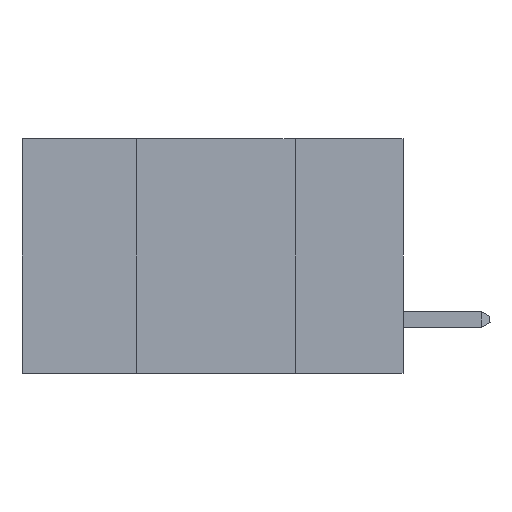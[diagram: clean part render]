
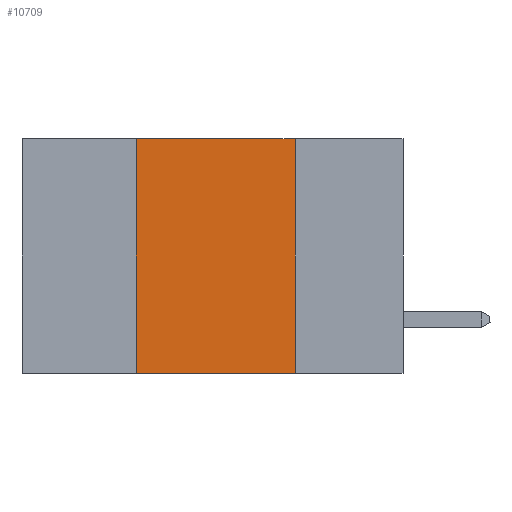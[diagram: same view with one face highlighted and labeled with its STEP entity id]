
A CAD part, left-side view. The second image highlights one B-rep face of the part: STEP entity #10709.
In plain terms, the highlighted planar face has unit normal (-1, 0, 0).
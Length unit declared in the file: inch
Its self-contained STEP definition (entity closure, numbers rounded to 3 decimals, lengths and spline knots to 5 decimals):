
#49 = VECTOR ( 'NONE', #16584, 39.37008 ) ;
#674 = CARTESIAN_POINT ( 'NONE',  ( 0., 0.42, -0.37 ) ) ;
#1449 = DIRECTION ( 'NONE',  ( 0., 0., -1. ) ) ;
#2698 = ORIENTED_EDGE ( 'NONE', *, *, #3617, .F. ) ;
#2763 = AXIS2_PLACEMENT_3D ( 'NONE', #7770, #7904, #1449 ) ;
#3161 = FACE_OUTER_BOUND ( 'NONE', #6307, .T. ) ;
#3617 = EDGE_CURVE ( 'NONE', #12747, #12285, #8369, .T. ) ;
#3653 = VECTOR ( 'NONE', #14696, 39.37008 ) ;
#5857 = CARTESIAN_POINT ( 'NONE',  ( 0., 0.17, 0. ) ) ;
#6307 = EDGE_LOOP ( 'NONE', ( #6329, #19401, #2698, #15257 ) ) ;
#6329 = ORIENTED_EDGE ( 'NONE', *, *, #15482, .F. ) ;
#6405 = CARTESIAN_POINT ( 'NONE',  ( 0., 0.6, 0. ) ) ;
#6597 = DIRECTION ( 'NONE',  ( 0., -1., 0. ) ) ;
#6686 = CARTESIAN_POINT ( 'NONE',  ( 0., 0.42, 0. ) ) ;
#7086 = CARTESIAN_POINT ( 'NONE',  ( 0., 0.17, -0.37 ) ) ;
#7698 = VECTOR ( 'NONE', #16196, 39.37008 ) ;
#7770 = CARTESIAN_POINT ( 'NONE',  ( 0., 0.6, 0. ) ) ;
#7904 = DIRECTION ( 'NONE',  ( 1., 0., 0. ) ) ;
#7906 = EDGE_CURVE ( 'NONE', #12285, #15036, #14683, .T. ) ;
#8369 = LINE ( 'NONE', #6686, #3653 ) ;
#10099 = LINE ( 'NONE', #11348, #17526 ) ;
#10709 = ADVANCED_FACE ( 'NONE', ( #3161 ), #20320, .F. ) ;
#11348 = CARTESIAN_POINT ( 'NONE',  ( 0., 0.6, -0.37 ) ) ;
#12285 = VERTEX_POINT ( 'NONE', #19545 ) ;
#12747 = VERTEX_POINT ( 'NONE', #674 ) ;
#13448 = VERTEX_POINT ( 'NONE', #7086 ) ;
#14511 = LINE ( 'NONE', #18129, #49 ) ;
#14683 = LINE ( 'NONE', #6405, #7698 ) ;
#14696 = DIRECTION ( 'NONE',  ( 0., 0., 1. ) ) ;
#15036 = VERTEX_POINT ( 'NONE', #5857 ) ;
#15257 = ORIENTED_EDGE ( 'NONE', *, *, #20266, .T. ) ;
#15482 = EDGE_CURVE ( 'NONE', #15036, #13448, #14511, .T. ) ;
#16196 = DIRECTION ( 'NONE',  ( 0., -1., 0. ) ) ;
#16584 = DIRECTION ( 'NONE',  ( 0., 0., -1. ) ) ;
#17526 = VECTOR ( 'NONE', #6597, 39.37008 ) ;
#18129 = CARTESIAN_POINT ( 'NONE',  ( 0., 0.17, 0. ) ) ;
#19401 = ORIENTED_EDGE ( 'NONE', *, *, #7906, .F. ) ;
#19545 = CARTESIAN_POINT ( 'NONE',  ( 0., 0.42, 0. ) ) ;
#20266 = EDGE_CURVE ( 'NONE', #12747, #13448, #10099, .T. ) ;
#20320 = PLANE ( 'NONE',  #2763 ) ;
